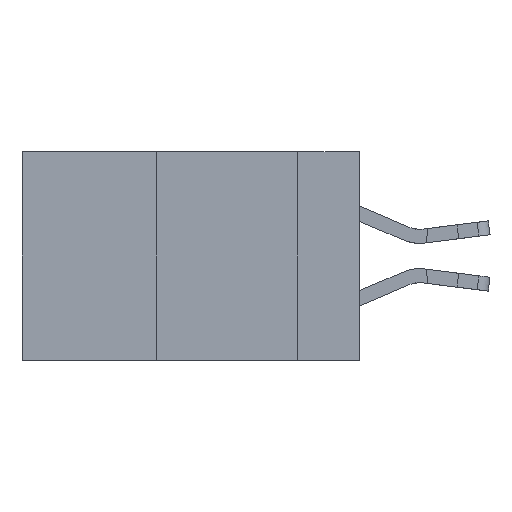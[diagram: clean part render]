
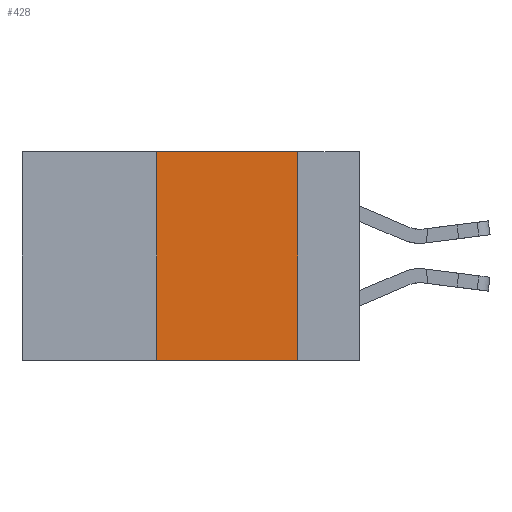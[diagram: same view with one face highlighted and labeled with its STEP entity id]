
A CAD part, left-side view. The second image highlights one B-rep face of the part: STEP entity #428.
In plain terms, the highlighted planar face has unit normal (-1, 0, 0).
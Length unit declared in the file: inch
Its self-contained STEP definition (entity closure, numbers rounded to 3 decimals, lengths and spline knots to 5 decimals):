
#428 = ADVANCED_FACE ( 'NONE', ( #15461 ), #7828, .F. ) ;
#1170 = VECTOR ( 'NONE', #18131, 39.37008 ) ;
#1780 = VERTEX_POINT ( 'NONE', #5578 ) ;
#1818 = LINE ( 'NONE', #15151, #7174 ) ;
#2177 = VERTEX_POINT ( 'NONE', #6557 ) ;
#3718 = EDGE_CURVE ( 'NONE', #1780, #2177, #21369, .T. ) ;
#5313 = EDGE_CURVE ( 'NONE', #17119, #1780, #23933, .T. ) ;
#5578 = CARTESIAN_POINT ( 'NONE',  ( 0., 0.11, 0. ) ) ;
#6159 = EDGE_CURVE ( 'NONE', #20080, #2177, #1818, .T. ) ;
#6557 = CARTESIAN_POINT ( 'NONE',  ( 0., 0.11, -0.37 ) ) ;
#7027 = EDGE_CURVE ( 'NONE', #20080, #17119, #27062, .T. ) ;
#7174 = VECTOR ( 'NONE', #21906, 39.37008 ) ;
#7828 = PLANE ( 'NONE',  #22717 ) ;
#9534 = ORIENTED_EDGE ( 'NONE', *, *, #3718, .F. ) ;
#13803 = CARTESIAN_POINT ( 'NONE',  ( 0., 0.6, 0. ) ) ;
#14229 = EDGE_LOOP ( 'NONE', ( #9534, #21359, #16850, #26273 ) ) ;
#15151 = CARTESIAN_POINT ( 'NONE',  ( 0., 0.6, -0.37 ) ) ;
#15461 = FACE_OUTER_BOUND ( 'NONE', #14229, .T. ) ;
#16807 = DIRECTION ( 'NONE',  ( 0., 0., 1. ) ) ;
#16850 = ORIENTED_EDGE ( 'NONE', *, *, #7027, .F. ) ;
#17119 = VERTEX_POINT ( 'NONE', #20369 ) ;
#18008 = VECTOR ( 'NONE', #16807, 39.37008 ) ;
#18131 = DIRECTION ( 'NONE',  ( 0., -1., 0. ) ) ;
#19599 = CARTESIAN_POINT ( 'NONE',  ( 0., 0.11, 0. ) ) ;
#19967 = DIRECTION ( 'NONE',  ( 0., 0., -1. ) ) ;
#20080 = VERTEX_POINT ( 'NONE', #21807 ) ;
#20369 = CARTESIAN_POINT ( 'NONE',  ( 0., 0.36, 0. ) ) ;
#20744 = CARTESIAN_POINT ( 'NONE',  ( 0., 0.6, 0. ) ) ;
#21074 = CARTESIAN_POINT ( 'NONE',  ( 0., 0.36, 0. ) ) ;
#21359 = ORIENTED_EDGE ( 'NONE', *, *, #5313, .F. ) ;
#21369 = LINE ( 'NONE', #19599, #22714 ) ;
#21807 = CARTESIAN_POINT ( 'NONE',  ( 0., 0.36, -0.37 ) ) ;
#21906 = DIRECTION ( 'NONE',  ( 0., -1., 0. ) ) ;
#22714 = VECTOR ( 'NONE', #19967, 39.37008 ) ;
#22717 = AXIS2_PLACEMENT_3D ( 'NONE', #20744, #24839, #25226 ) ;
#23933 = LINE ( 'NONE', #13803, #1170 ) ;
#24839 = DIRECTION ( 'NONE',  ( 1., 0., 0. ) ) ;
#25226 = DIRECTION ( 'NONE',  ( 0., 0., -1. ) ) ;
#26273 = ORIENTED_EDGE ( 'NONE', *, *, #6159, .T. ) ;
#27062 = LINE ( 'NONE', #21074, #18008 ) ;
